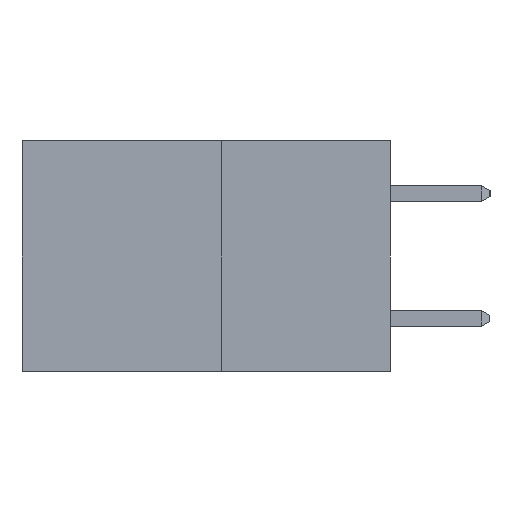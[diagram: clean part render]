
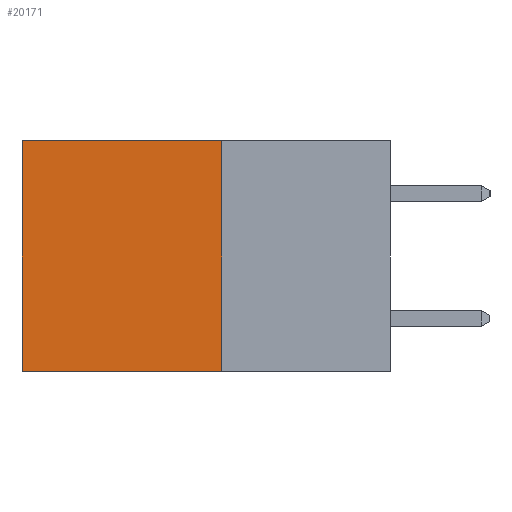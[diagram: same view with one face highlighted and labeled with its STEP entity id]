
A CAD part, left-side view. The second image highlights one B-rep face of the part: STEP entity #20171.
In plain terms, the highlighted planar face has unit normal (-1, 0, 0).
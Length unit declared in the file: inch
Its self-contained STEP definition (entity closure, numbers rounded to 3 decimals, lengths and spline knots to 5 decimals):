
#95 = DIRECTION ( 'NONE',  ( 0., 1., 0. ) ) ;
#269 = CARTESIAN_POINT ( 'NONE',  ( 0.277, 0.59, -0.37 ) ) ;
#295 = DIRECTION ( 'NONE',  ( 0., 0., -1. ) ) ;
#1960 = CARTESIAN_POINT ( 'NONE',  ( 0.277, 0.27, -0.37 ) ) ;
#3120 = CARTESIAN_POINT ( 'NONE',  ( 0.277, 0.27, -0.37 ) ) ;
#3357 = VERTEX_POINT ( 'NONE', #22258 ) ;
#4960 = DIRECTION ( 'NONE',  ( 0., 0., -1. ) ) ;
#5233 = EDGE_CURVE ( 'NONE', #3357, #18789, #13113, .T. ) ;
#5557 = EDGE_LOOP ( 'NONE', ( #13980, #14237, #14299, #14474 ) ) ;
#5772 = EDGE_CURVE ( 'NONE', #9197, #10784, #17371, .T. ) ;
#6317 = LINE ( 'NONE', #1960, #15435 ) ;
#6838 = DIRECTION ( 'NONE',  ( 0., 0., -1. ) ) ;
#6856 = CARTESIAN_POINT ( 'NONE',  ( 0.277, 0.27, -0.37 ) ) ;
#7136 = VECTOR ( 'NONE', #295, 39.37008 ) ;
#8077 = CARTESIAN_POINT ( 'NONE',  ( 0.277, 0.27, 0. ) ) ;
#8348 = CARTESIAN_POINT ( 'NONE',  ( 0.277, 0.59, 0. ) ) ;
#9197 = VERTEX_POINT ( 'NONE', #8348 ) ;
#9443 = VECTOR ( 'NONE', #6838, 39.37008 ) ;
#9668 = CARTESIAN_POINT ( 'NONE',  ( 0.277, 0.59, -0.37 ) ) ;
#9926 = DIRECTION ( 'NONE',  ( 0., 1., 0. ) ) ;
#10784 = VERTEX_POINT ( 'NONE', #9668 ) ;
#11336 = EDGE_CURVE ( 'NONE', #18789, #10784, #6317, .T. ) ;
#13113 = LINE ( 'NONE', #6856, #9443 ) ;
#13955 = EDGE_CURVE ( 'NONE', #3357, #9197, #17557, .T. ) ;
#13980 = ORIENTED_EDGE ( 'NONE', *, *, #5772, .T. ) ;
#13999 = FACE_OUTER_BOUND ( 'NONE', #5557, .T. ) ;
#14237 = ORIENTED_EDGE ( 'NONE', *, *, #11336, .F. ) ;
#14299 = ORIENTED_EDGE ( 'NONE', *, *, #5233, .F. ) ;
#14474 = ORIENTED_EDGE ( 'NONE', *, *, #13955, .T. ) ;
#15435 = VECTOR ( 'NONE', #95, 39.37008 ) ;
#15895 = DIRECTION ( 'NONE',  ( 1., 0., 0. ) ) ;
#17371 = LINE ( 'NONE', #269, #7136 ) ;
#17557 = LINE ( 'NONE', #8077, #23386 ) ;
#18706 = AXIS2_PLACEMENT_3D ( 'NONE', #3120, #15895, #4960 ) ;
#18789 = VERTEX_POINT ( 'NONE', #22152 ) ;
#20171 = ADVANCED_FACE ( 'NONE', ( #13999 ), #22987, .F. ) ;
#22152 = CARTESIAN_POINT ( 'NONE',  ( 0.277, 0.27, -0.37 ) ) ;
#22258 = CARTESIAN_POINT ( 'NONE',  ( 0.277, 0.27, 0. ) ) ;
#22987 = PLANE ( 'NONE',  #18706 ) ;
#23386 = VECTOR ( 'NONE', #9926, 39.37008 ) ;
